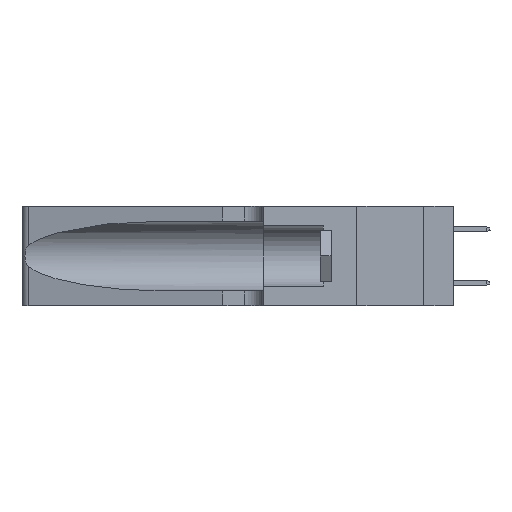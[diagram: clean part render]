
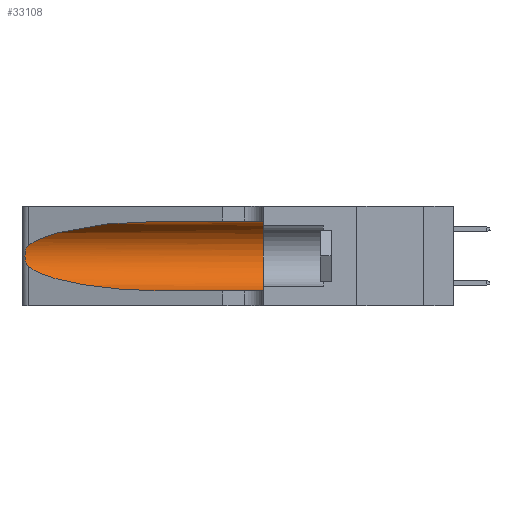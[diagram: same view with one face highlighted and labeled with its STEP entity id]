
A CAD part, left-side view. The second image highlights one B-rep face of the part: STEP entity #33108.
In plain terms, the highlighted cylindrical face has radius 3.308 mm (diameter 6.617 mm), a partial arc.
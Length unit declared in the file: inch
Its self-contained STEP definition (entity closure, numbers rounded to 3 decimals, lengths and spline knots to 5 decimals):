
#673 = CARTESIAN_POINT ( 'NONE',  ( 0.1305, 0.72297, 0.05475 ) ) ;
#1101 = CARTESIAN_POINT ( 'NONE',  ( 0.25555, 1.22993, 0.14849 ) ) ;
#1811 = CARTESIAN_POINT ( 'NONE',  ( 0.25787, 1.23484, 0.2124 ) ) ;
#1889 = CARTESIAN_POINT ( 'NONE',  ( 0.25487, 1.22718, 0.22369 ) ) ;
#4424 = CARTESIAN_POINT ( 'NONE',  ( 0.26017, 1.23833, 0.17102 ) ) ;
#5098 = CARTESIAN_POINT ( 'NONE',  ( 0.1305, 0.72297, 0.05475 ) ) ;
#5532 = CARTESIAN_POINT ( 'NONE',  ( 0.2373, 1.15595, 0.28018 ) ) ;
#6251 = ORIENTED_EDGE ( 'NONE', *, *, #22222, .T. ) ;
#6262 = EDGE_LOOP ( 'NONE', ( #6251, #9034, #11081, #45514, #36549, #12639 ) ) ;
#7674 = EDGE_CURVE ( 'NONE', #43067, #18983, #9931, .T. ) ;
#7725 =( BOUNDED_CURVE ( )  B_SPLINE_CURVE ( 3, ( #38199, #27009, #5532, #19595 ),
 .UNSPECIFIED., .F., .F. ) 
 B_SPLINE_CURVE_WITH_KNOTS ( ( 4, 4 ),
 ( 1.5708, 2.84003 ),
 .UNSPECIFIED. ) 
 CURVE ( )  GEOMETRIC_REPRESENTATION_ITEM ( )  RATIONAL_B_SPLINE_CURVE ( ( 1., 0.87, 0.87, 1. ) ) 
 REPRESENTATION_ITEM ( '' )  );
#8120 = CYLINDRICAL_SURFACE ( 'NONE', #36668, 0.13025 ) ;
#8121 = CARTESIAN_POINT ( 'NONE',  ( 0.2373, 1.15595, 0.08982 ) ) ;
#8253 = VERTEX_POINT ( 'NONE', #42715 ) ;
#8869 = VERTEX_POINT ( 'NONE', #14286 ) ;
#8924 = CARTESIAN_POINT ( 'NONE',  ( 0.25487, 1.22718, 0.22369 ) ) ;
#9034 = ORIENTED_EDGE ( 'NONE', *, *, #7674, .T. ) ;
#9931 = B_SPLINE_CURVE_WITH_KNOTS ( 'NONE', 3,
 ( #8924, #37052, #45172, #1811, #19182, #22530, #15374, #12520, #4424, #11811, #33728, #33492, #1101, #27069 ),
 .UNSPECIFIED., .F., .F.,
 ( 4, 2, 2, 2, 2, 2, 4 ),
 ( 0., 0.00027, 0.00053, 0.00107, 0.0016, 0.00187, 0.00214 ),
 .UNSPECIFIED. ) ;
#10925 = CARTESIAN_POINT ( 'NONE',  ( 0.18966, 0.96281, 0.05475 ) ) ;
#11081 = ORIENTED_EDGE ( 'NONE', *, *, #19318, .T. ) ;
#11708 = CARTESIAN_POINT ( 'NONE',  ( 0.1305, 1.61858, 0.185 ) ) ;
#11811 = CARTESIAN_POINT ( 'NONE',  ( 0.25856, 1.23593, 0.16098 ) ) ;
#12520 = CARTESIAN_POINT ( 'NONE',  ( 0.26075, 1.23896, 0.178 ) ) ;
#12639 = ORIENTED_EDGE ( 'NONE', *, *, #17609, .F. ) ;
#13638 = VERTEX_POINT ( 'NONE', #5098 ) ;
#14121 = CARTESIAN_POINT ( 'NONE',  ( 0.1305, 1.61858, 0.05475 ) ) ;
#14286 = CARTESIAN_POINT ( 'NONE',  ( 0.1305, 0.72297, 0.31525 ) ) ;
#15374 = CARTESIAN_POINT ( 'NONE',  ( 0.26075, 1.23896, 0.19203 ) ) ;
#15522 = CARTESIAN_POINT ( 'NONE',  ( 0.25487, 1.22718, 0.14631 ) ) ;
#15562 = VECTOR ( 'NONE', #25504, 39.37008 ) ;
#15624 = EDGE_CURVE ( 'NONE', #13638, #8253, #43191, .T. ) ;
#16947 = DIRECTION ( 'NONE',  ( 0., -1., 0. ) ) ;
#17609 = EDGE_CURVE ( 'NONE', #8869, #27056, #29783, .T. ) ;
#18983 = VERTEX_POINT ( 'NONE', #15522 ) ;
#19182 = CARTESIAN_POINT ( 'NONE',  ( 0.25854, 1.2359, 0.20912 ) ) ;
#19318 = EDGE_CURVE ( 'NONE', #18983, #13638, #35153, .T. ) ;
#19595 = CARTESIAN_POINT ( 'NONE',  ( 0.25487, 1.22718, 0.22369 ) ) ;
#22222 = EDGE_CURVE ( 'NONE', #8869, #43067, #7725, .T. ) ;
#22530 = CARTESIAN_POINT ( 'NONE',  ( 0.26018, 1.23835, 0.19895 ) ) ;
#22672 = DIRECTION ( 'NONE',  ( 0., -1., 0. ) ) ;
#24616 = VECTOR ( 'NONE', #16947, 39.37008 ) ;
#25504 = DIRECTION ( 'NONE',  ( 0., -1., 0. ) ) ;
#26260 = FACE_OUTER_BOUND ( 'NONE', #6262, .T. ) ;
#27009 = CARTESIAN_POINT ( 'NONE',  ( 0.18966, 0.96281, 0.31525 ) ) ;
#27056 = VERTEX_POINT ( 'NONE', #40339 ) ;
#27069 = CARTESIAN_POINT ( 'NONE',  ( 0.25487, 1.22718, 0.14631 ) ) ;
#27538 = CIRCLE ( 'NONE', #46545, 0.13025 ) ;
#28556 = DIRECTION ( 'NONE',  ( 0., 1., 0. ) ) ;
#29783 = LINE ( 'NONE', #35989, #15562 ) ;
#33108 = ADVANCED_FACE ( 'NONE', ( #26260 ), #8120, .F. ) ;
#33492 = CARTESIAN_POINT ( 'NONE',  ( 0.25639, 1.23186, 0.15144 ) ) ;
#33728 = CARTESIAN_POINT ( 'NONE',  ( 0.25789, 1.23486, 0.15765 ) ) ;
#35153 =( BOUNDED_CURVE ( )  B_SPLINE_CURVE ( 3, ( #37090, #8121, #10925, #673 ),
 .UNSPECIFIED., .F., .F. ) 
 B_SPLINE_CURVE_WITH_KNOTS ( ( 4, 4 ),
 ( 3.44316, 4.71239 ),
 .UNSPECIFIED. ) 
 CURVE ( )  GEOMETRIC_REPRESENTATION_ITEM ( )  RATIONAL_B_SPLINE_CURVE ( ( 1., 0.87, 0.87, 1. ) ) 
 REPRESENTATION_ITEM ( '' )  );
#35229 = EDGE_CURVE ( 'NONE', #27056, #8253, #27538, .T. ) ;
#35989 = CARTESIAN_POINT ( 'NONE',  ( 0.1305, 1.61858, 0.31525 ) ) ;
#36549 = ORIENTED_EDGE ( 'NONE', *, *, #35229, .F. ) ;
#36668 = AXIS2_PLACEMENT_3D ( 'NONE', #11708, #22672, #40073 ) ;
#37052 = CARTESIAN_POINT ( 'NONE',  ( 0.25555, 1.22994, 0.2215 ) ) ;
#37090 = CARTESIAN_POINT ( 'NONE',  ( 0.25487, 1.22718, 0.14631 ) ) ;
#38199 = CARTESIAN_POINT ( 'NONE',  ( 0.1305, 0.72297, 0.31525 ) ) ;
#39273 = CARTESIAN_POINT ( 'NONE',  ( 0.1305, 0.35, 0.185 ) ) ;
#40073 = DIRECTION ( 'NONE',  ( 0., 0., -1. ) ) ;
#40339 = CARTESIAN_POINT ( 'NONE',  ( 0.1305, 0.35, 0.31525 ) ) ;
#42715 = CARTESIAN_POINT ( 'NONE',  ( 0.1305, 0.35, 0.05475 ) ) ;
#43067 = VERTEX_POINT ( 'NONE', #1889 ) ;
#43082 = DIRECTION ( 'NONE',  ( 0., 0., 1. ) ) ;
#43191 = LINE ( 'NONE', #14121, #24616 ) ;
#45172 = CARTESIAN_POINT ( 'NONE',  ( 0.25639, 1.23184, 0.21858 ) ) ;
#45514 = ORIENTED_EDGE ( 'NONE', *, *, #15624, .T. ) ;
#46545 = AXIS2_PLACEMENT_3D ( 'NONE', #39273, #28556, #43082 ) ;
